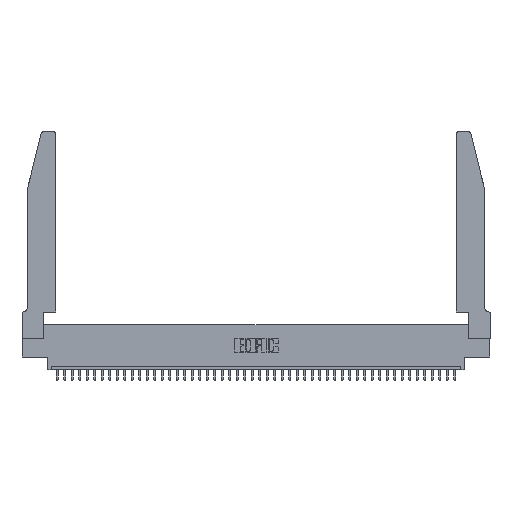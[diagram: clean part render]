
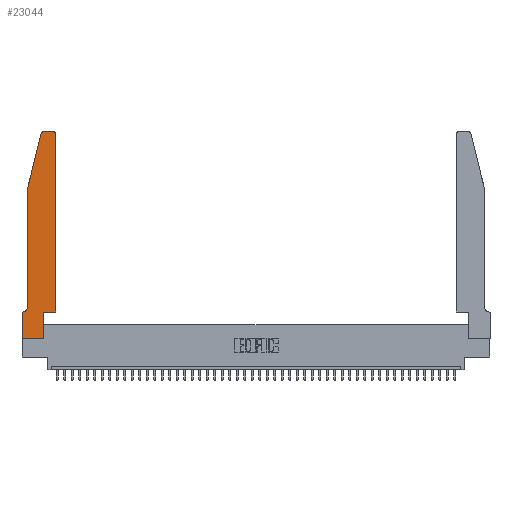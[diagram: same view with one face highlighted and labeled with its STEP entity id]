
A CAD part, top view. The second image highlights one B-rep face of the part: STEP entity #23044.
In plain terms, the highlighted planar face has unit normal (0, 0, 1).
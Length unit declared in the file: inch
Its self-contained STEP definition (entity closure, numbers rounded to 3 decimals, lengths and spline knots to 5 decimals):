
#154 = CIRCLE ( 'NONE', #798, 0.03 ) ;
#798 = AXIS2_PLACEMENT_3D ( 'NONE', #36345, #36491, #6152 ) ;
#928 = VERTEX_POINT ( 'NONE', #8293 ) ;
#1663 = AXIS2_PLACEMENT_3D ( 'NONE', #21702, #27512, #25124 ) ;
#2140 = PLANE ( 'NONE',  #35585 ) ;
#3120 = EDGE_CURVE ( 'NONE', #9452, #928, #8944, .T. ) ;
#3945 = DIRECTION ( 'NONE',  ( 0., 0., 1. ) ) ;
#4161 = EDGE_LOOP ( 'NONE', ( #8455, #37540, #39690, #28803, #7923, #10109, #10228, #15324, #29225, #20611, #42403, #12960 ) ) ;
#4812 = VECTOR ( 'NONE', #18918, 39.37008 ) ;
#5223 = DIRECTION ( 'NONE',  ( -0.239, -0.971, 0. ) ) ;
#5405 = DIRECTION ( 'NONE',  ( 1., 0., 0. ) ) ;
#5790 = CARTESIAN_POINT ( 'NONE',  ( 0.25487, 2.72718, 0.37 ) ) ;
#6152 = DIRECTION ( 'NONE',  ( 1., 0., 0. ) ) ;
#6269 = CARTESIAN_POINT ( 'NONE',  ( 0.0755, 2., 0.37 ) ) ;
#6500 = VECTOR ( 'NONE', #40095, 39.37008 ) ;
#6860 = EDGE_CURVE ( 'NONE', #22675, #9452, #26172, .T. ) ;
#7338 = CARTESIAN_POINT ( 'NONE',  ( 0., 0., 0.37 ) ) ;
#7660 = CARTESIAN_POINT ( 'NONE',  ( 0.4505, 0.35, 0.37 ) ) ;
#7923 = ORIENTED_EDGE ( 'NONE', *, *, #6860, .T. ) ;
#8293 = CARTESIAN_POINT ( 'NONE',  ( 0., 0.35, 0.37 ) ) ;
#8455 = ORIENTED_EDGE ( 'NONE', *, *, #35729, .T. ) ;
#8944 = LINE ( 'NONE', #19857, #10494 ) ;
#9452 = VERTEX_POINT ( 'NONE', #19955 ) ;
#10109 = ORIENTED_EDGE ( 'NONE', *, *, #3120, .T. ) ;
#10228 = ORIENTED_EDGE ( 'NONE', *, *, #25272, .T. ) ;
#10356 = LINE ( 'NONE', #7338, #30036 ) ;
#10494 = VECTOR ( 'NONE', #30290, 39.37008 ) ;
#11461 = CARTESIAN_POINT ( 'NONE',  ( 0., 0., 0.37 ) ) ;
#12217 = CARTESIAN_POINT ( 'NONE',  ( 0.2605, 2.75, 0.37 ) ) ;
#12960 = ORIENTED_EDGE ( 'NONE', *, *, #26961, .T. ) ;
#13841 = DIRECTION ( 'NONE',  ( 0., -1., 0. ) ) ;
#14738 = LINE ( 'NONE', #15536, #22240 ) ;
#15324 = ORIENTED_EDGE ( 'NONE', *, *, #34692, .T. ) ;
#15536 = CARTESIAN_POINT ( 'NONE',  ( 0.0755, 2., 0.37 ) ) ;
#16817 = CARTESIAN_POINT ( 'NONE',  ( 0.0755, 0.42, 0.37 ) ) ;
#16963 = LINE ( 'NONE', #12217, #20145 ) ;
#17330 = EDGE_CURVE ( 'NONE', #21884, #20276, #14738, .T. ) ;
#17353 = VERTEX_POINT ( 'NONE', #32331 ) ;
#17698 = DIRECTION ( 'NONE',  ( 0., 1., 0. ) ) ;
#18104 = VERTEX_POINT ( 'NONE', #31923 ) ;
#18278 = VERTEX_POINT ( 'NONE', #29402 ) ;
#18666 = CARTESIAN_POINT ( 'NONE',  ( 0., 0.35, 0.37 ) ) ;
#18918 = DIRECTION ( 'NONE',  ( 0., 1., 0. ) ) ;
#19636 = VERTEX_POINT ( 'NONE', #11461 ) ;
#19724 = CARTESIAN_POINT ( 'NONE',  ( 0.4505, 0.35, 0.37 ) ) ;
#19757 = EDGE_CURVE ( 'NONE', #18104, #40995, #20426, .T. ) ;
#19857 = CARTESIAN_POINT ( 'NONE',  ( 0.0755, 0.35, 0.37 ) ) ;
#19955 = CARTESIAN_POINT ( 'NONE',  ( 0.0055, 0.35, 0.37 ) ) ;
#20145 = VECTOR ( 'NONE', #39389, 39.37008 ) ;
#20276 = VERTEX_POINT ( 'NONE', #35881 ) ;
#20426 = LINE ( 'NONE', #19724, #37412 ) ;
#20611 = ORIENTED_EDGE ( 'NONE', *, *, #19757, .T. ) ;
#21702 = CARTESIAN_POINT ( 'NONE',  ( 0.0055, 0.42, 0.37 ) ) ;
#21884 = VERTEX_POINT ( 'NONE', #5790 ) ;
#22240 = VECTOR ( 'NONE', #5223, 39.37008 ) ;
#22429 = CIRCLE ( 'NONE', #34368, 0.03 ) ;
#22675 = VERTEX_POINT ( 'NONE', #16817 ) ;
#23044 = ADVANCED_FACE ( 'NONE', ( #40831 ), #2140, .T. ) ;
#23441 = DIRECTION ( 'NONE',  ( 0., -1., 0. ) ) ;
#23534 = CARTESIAN_POINT ( 'NONE',  ( 0.4205, 2.75, 0.37 ) ) ;
#24230 = CARTESIAN_POINT ( 'NONE',  ( 0.284, 2.72, 0.37 ) ) ;
#24750 = EDGE_CURVE ( 'NONE', #29835, #18104, #25820, .T. ) ;
#24790 = DIRECTION ( 'NONE',  ( 1., 0., 0. ) ) ;
#24977 = VECTOR ( 'NONE', #23441, 39.37008 ) ;
#25124 = DIRECTION ( 'NONE',  ( -1., 0., 0. ) ) ;
#25272 = EDGE_CURVE ( 'NONE', #928, #19636, #10356, .T. ) ;
#25820 = LINE ( 'NONE', #31238, #41728 ) ;
#26172 = CIRCLE ( 'NONE', #1663, 0.07 ) ;
#26961 = EDGE_CURVE ( 'NONE', #18278, #43788, #154, .T. ) ;
#27512 = DIRECTION ( 'NONE',  ( 0., 0., -1. ) ) ;
#28803 = ORIENTED_EDGE ( 'NONE', *, *, #43177, .T. ) ;
#29225 = ORIENTED_EDGE ( 'NONE', *, *, #24750, .T. ) ;
#29402 = CARTESIAN_POINT ( 'NONE',  ( 0.4505, 2.72, 0.37 ) ) ;
#29835 = VERTEX_POINT ( 'NONE', #40325 ) ;
#30036 = VECTOR ( 'NONE', #13841, 39.37008 ) ;
#30290 = DIRECTION ( 'NONE',  ( -1., 0., 0. ) ) ;
#30318 = CARTESIAN_POINT ( 'NONE',  ( 0., 0., 0.37 ) ) ;
#31238 = CARTESIAN_POINT ( 'NONE',  ( 0.2865, 0.35, 0.37 ) ) ;
#31923 = CARTESIAN_POINT ( 'NONE',  ( 0.2865, 0.35, 0.37 ) ) ;
#32331 = CARTESIAN_POINT ( 'NONE',  ( 0.284, 2.75, 0.37 ) ) ;
#34368 = AXIS2_PLACEMENT_3D ( 'NONE', #24230, #3945, #37299 ) ;
#34692 = EDGE_CURVE ( 'NONE', #19636, #29835, #42016, .T. ) ;
#35020 = LINE ( 'NONE', #39288, #4812 ) ;
#35267 = EDGE_CURVE ( 'NONE', #40995, #18278, #35020, .T. ) ;
#35585 = AXIS2_PLACEMENT_3D ( 'NONE', #18666, #39167, #5405 ) ;
#35729 = EDGE_CURVE ( 'NONE', #43788, #17353, #16963, .T. ) ;
#35881 = CARTESIAN_POINT ( 'NONE',  ( 0.0755, 2., 0.37 ) ) ;
#36345 = CARTESIAN_POINT ( 'NONE',  ( 0.4205, 2.72, 0.37 ) ) ;
#36491 = DIRECTION ( 'NONE',  ( 0., 0., 1. ) ) ;
#37299 = DIRECTION ( 'NONE',  ( 1., 0., 0. ) ) ;
#37412 = VECTOR ( 'NONE', #24790, 39.37008 ) ;
#37540 = ORIENTED_EDGE ( 'NONE', *, *, #41367, .T. ) ;
#39167 = DIRECTION ( 'NONE',  ( 0., 0., 1. ) ) ;
#39288 = CARTESIAN_POINT ( 'NONE',  ( 0.4505, 0.35, 0.37 ) ) ;
#39389 = DIRECTION ( 'NONE',  ( -1., 0., 0. ) ) ;
#39690 = ORIENTED_EDGE ( 'NONE', *, *, #17330, .T. ) ;
#40095 = DIRECTION ( 'NONE',  ( 1., 0., 0. ) ) ;
#40325 = CARTESIAN_POINT ( 'NONE',  ( 0.2865, 0., 0.37 ) ) ;
#40831 = FACE_OUTER_BOUND ( 'NONE', #4161, .T. ) ;
#40995 = VERTEX_POINT ( 'NONE', #7660 ) ;
#41367 = EDGE_CURVE ( 'NONE', #17353, #21884, #22429, .T. ) ;
#41728 = VECTOR ( 'NONE', #17698, 39.37008 ) ;
#42016 = LINE ( 'NONE', #30318, #6500 ) ;
#42403 = ORIENTED_EDGE ( 'NONE', *, *, #35267, .T. ) ;
#43177 = EDGE_CURVE ( 'NONE', #20276, #22675, #43565, .T. ) ;
#43565 = LINE ( 'NONE', #6269, #24977 ) ;
#43788 = VERTEX_POINT ( 'NONE', #23534 ) ;
